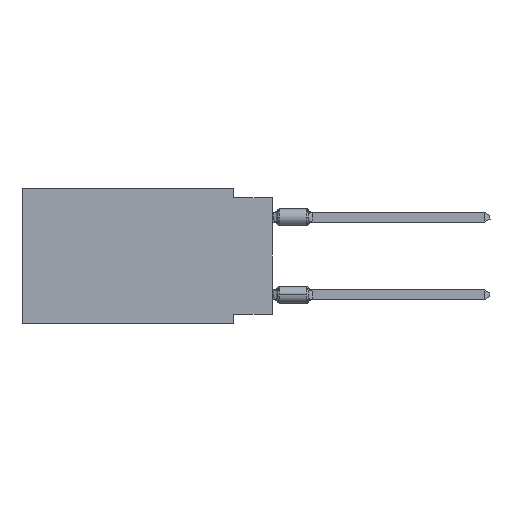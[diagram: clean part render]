
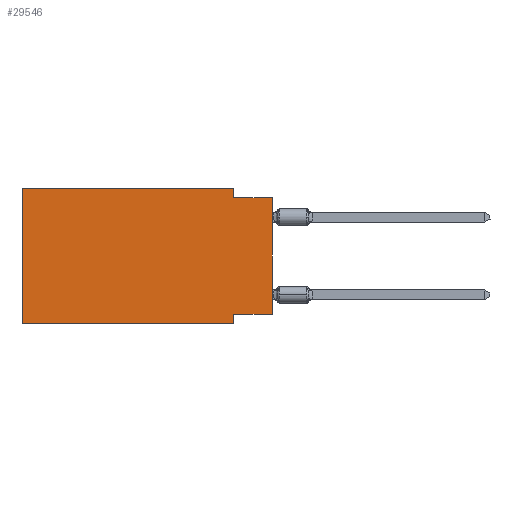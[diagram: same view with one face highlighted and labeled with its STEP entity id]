
A CAD part, left-side view. The second image highlights one B-rep face of the part: STEP entity #29546.
In plain terms, the highlighted planar face has unit normal (-1, 0, 0).
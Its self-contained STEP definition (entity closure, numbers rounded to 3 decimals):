
#1215 = LINE ( 'NONE', #8433, #46561 ) ;
#1464 = ORIENTED_EDGE ( 'NONE', *, *, #28935, .F. ) ;
#3232 = DIRECTION ( 'NONE',  ( 0., 0., -1. ) ) ;
#3606 = DIRECTION ( 'NONE',  ( 0., 0., 1. ) ) ;
#4085 = ORIENTED_EDGE ( 'NONE', *, *, #48718, .F. ) ;
#4970 = ORIENTED_EDGE ( 'NONE', *, *, #23083, .F. ) ;
#5858 = LINE ( 'NONE', #43329, #19819 ) ;
#6560 = CARTESIAN_POINT ( 'NONE',  ( 0., 0., -0.635 ) ) ;
#6733 = LINE ( 'NONE', #10936, #49045 ) ;
#6999 = DIRECTION ( 'NONE',  ( 1., 0., 0. ) ) ;
#7054 = EDGE_CURVE ( 'NONE', #28729, #28631, #40530, .T. ) ;
#7069 = DIRECTION ( 'NONE',  ( 0., -1., 0. ) ) ;
#8433 = CARTESIAN_POINT ( 'NONE',  ( 0., 0., -0.635 ) ) ;
#8615 = ORIENTED_EDGE ( 'NONE', *, *, #36247, .F. ) ;
#8917 = VECTOR ( 'NONE', #3606, 1000. ) ;
#10755 = EDGE_LOOP ( 'NONE', ( #40109, #4970, #8615, #42763, #30784, #31009, #4085, #1464 ) ) ;
#10936 = CARTESIAN_POINT ( 'NONE',  ( 0., 2.54, -8.89 ) ) ;
#11292 = CARTESIAN_POINT ( 'NONE',  ( 0., 0., 0. ) ) ;
#11790 = LINE ( 'NONE', #11292, #8917 ) ;
#12093 = CARTESIAN_POINT ( 'NONE',  ( 0., 2.54, -8.255 ) ) ;
#12454 = CARTESIAN_POINT ( 'NONE',  ( 0., 2.54, -8.89 ) ) ;
#14695 = VERTEX_POINT ( 'NONE', #12093 ) ;
#15161 = EDGE_CURVE ( 'NONE', #40446, #27391, #11790, .T. ) ;
#15317 = VECTOR ( 'NONE', #7069, 1000. ) ;
#15458 = DIRECTION ( 'NONE',  ( 0., -1., 0. ) ) ;
#15921 = VERTEX_POINT ( 'NONE', #41969 ) ;
#16714 = EDGE_CURVE ( 'NONE', #28631, #15921, #37334, .T. ) ;
#18213 = LINE ( 'NONE', #18448, #40248 ) ;
#18405 = DIRECTION ( 'NONE',  ( 0., 0., -1. ) ) ;
#18448 = CARTESIAN_POINT ( 'NONE',  ( 0., 16.383, -8.89 ) ) ;
#18523 = CARTESIAN_POINT ( 'NONE',  ( 0., 16.383, 0. ) ) ;
#19819 = VECTOR ( 'NONE', #44292, 1000. ) ;
#20350 = LINE ( 'NONE', #31253, #43759 ) ;
#21897 = FACE_OUTER_BOUND ( 'NONE', #10755, .T. ) ;
#22926 = VERTEX_POINT ( 'NONE', #25157 ) ;
#23083 = EDGE_CURVE ( 'NONE', #22926, #27391, #1215, .T. ) ;
#23483 = EDGE_CURVE ( 'NONE', #28729, #30833, #18213, .T. ) ;
#23572 = DIRECTION ( 'NONE',  ( 0., 0., -1. ) ) ;
#25157 = CARTESIAN_POINT ( 'NONE',  ( 0., 2.54, -0.635 ) ) ;
#27391 = VERTEX_POINT ( 'NONE', #6560 ) ;
#28631 = VERTEX_POINT ( 'NONE', #18523 ) ;
#28729 = VERTEX_POINT ( 'NONE', #37862 ) ;
#28885 = DIRECTION ( 'NONE',  ( 0., 0., 1. ) ) ;
#28935 = EDGE_CURVE ( 'NONE', #40446, #14695, #5858, .T. ) ;
#29546 = ADVANCED_FACE ( 'NONE', ( #21897 ), #37028, .F. ) ;
#30784 = ORIENTED_EDGE ( 'NONE', *, *, #7054, .F. ) ;
#30833 = VERTEX_POINT ( 'NONE', #12454 ) ;
#31009 = ORIENTED_EDGE ( 'NONE', *, *, #23483, .T. ) ;
#31253 = CARTESIAN_POINT ( 'NONE',  ( 0., 2.54, 0. ) ) ;
#36247 = EDGE_CURVE ( 'NONE', #15921, #22926, #20350, .T. ) ;
#36507 = AXIS2_PLACEMENT_3D ( 'NONE', #44710, #6999, #18405 ) ;
#37028 = PLANE ( 'NONE',  #36507 ) ;
#37334 = LINE ( 'NONE', #41295, #15317 ) ;
#37862 = CARTESIAN_POINT ( 'NONE',  ( 0., 16.383, -8.89 ) ) ;
#40109 = ORIENTED_EDGE ( 'NONE', *, *, #15161, .T. ) ;
#40248 = VECTOR ( 'NONE', #15458, 1000. ) ;
#40446 = VERTEX_POINT ( 'NONE', #48597 ) ;
#40530 = LINE ( 'NONE', #44493, #41554 ) ;
#41295 = CARTESIAN_POINT ( 'NONE',  ( 0., 16.383, 0. ) ) ;
#41554 = VECTOR ( 'NONE', #28885, 1000. ) ;
#41969 = CARTESIAN_POINT ( 'NONE',  ( 0., 2.54, 0. ) ) ;
#42665 = DIRECTION ( 'NONE',  ( 0., -1., 0. ) ) ;
#42763 = ORIENTED_EDGE ( 'NONE', *, *, #16714, .F. ) ;
#43329 = CARTESIAN_POINT ( 'NONE',  ( 0., 0., -8.255 ) ) ;
#43759 = VECTOR ( 'NONE', #23572, 1000. ) ;
#44292 = DIRECTION ( 'NONE',  ( 0., 1., 0. ) ) ;
#44493 = CARTESIAN_POINT ( 'NONE',  ( 0., 16.383, 0. ) ) ;
#44710 = CARTESIAN_POINT ( 'NONE',  ( 0., 16.383, 0. ) ) ;
#46561 = VECTOR ( 'NONE', #42665, 1000. ) ;
#48597 = CARTESIAN_POINT ( 'NONE',  ( 0., 0., -8.255 ) ) ;
#48718 = EDGE_CURVE ( 'NONE', #14695, #30833, #6733, .T. ) ;
#49045 = VECTOR ( 'NONE', #3232, 1000. ) ;
